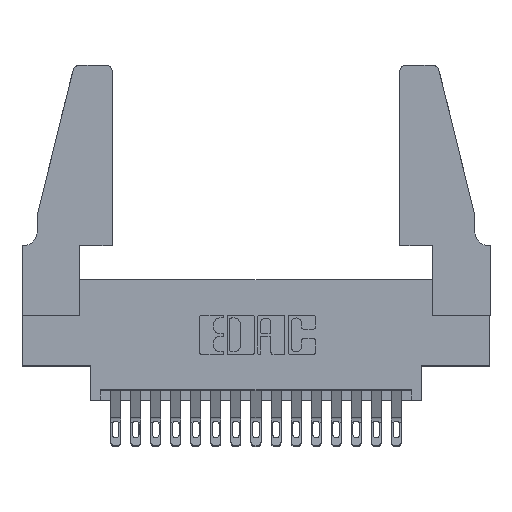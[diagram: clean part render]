
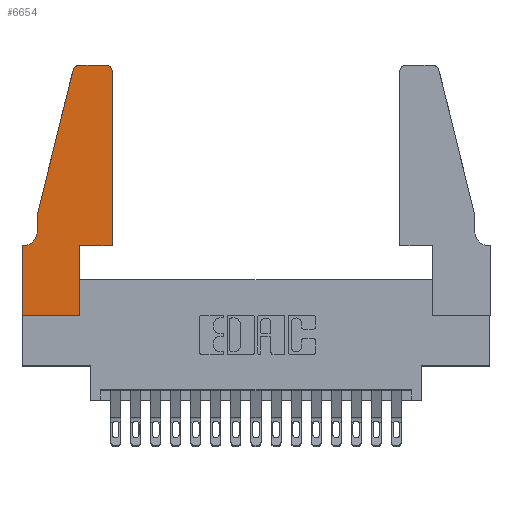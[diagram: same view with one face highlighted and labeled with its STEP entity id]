
A CAD part, top view. The second image highlights one B-rep face of the part: STEP entity #6654.
In plain terms, the highlighted planar face has unit normal (0, 0, 1).
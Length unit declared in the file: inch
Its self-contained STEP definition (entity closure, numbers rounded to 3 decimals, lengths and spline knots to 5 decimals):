
#56 = EDGE_CURVE ( 'NONE', #10528, #17273, #4938, .T. ) ;
#366 = ORIENTED_EDGE ( 'NONE', *, *, #56, .T. ) ;
#660 = CARTESIAN_POINT ( 'NONE',  ( 0.0055, 0.35, 0.37 ) ) ;
#1208 = DIRECTION ( 'NONE',  ( 1., 0., 0. ) ) ;
#1233 = VERTEX_POINT ( 'NONE', #3047 ) ;
#1381 = CARTESIAN_POINT ( 'NONE',  ( 0., 0., 0.37 ) ) ;
#1388 = LINE ( 'NONE', #16381, #8575 ) ;
#1417 = DIRECTION ( 'NONE',  ( -1., 0., 0. ) ) ;
#1424 = EDGE_CURVE ( 'NONE', #9109, #14748, #5887, .T. ) ;
#1630 = DIRECTION ( 'NONE',  ( -1., 0., 0. ) ) ;
#1920 = DIRECTION ( 'NONE',  ( -0.239, -0.971, 0. ) ) ;
#2594 = DIRECTION ( 'NONE',  ( 0., 1., 0. ) ) ;
#2750 = DIRECTION ( 'NONE',  ( 1., 0., 0. ) ) ;
#2854 = CIRCLE ( 'NONE', #13362, 0.03 ) ;
#3047 = CARTESIAN_POINT ( 'NONE',  ( 0.4505, 0.35, 0.37 ) ) ;
#3548 = EDGE_CURVE ( 'NONE', #12391, #12999, #15243, .T. ) ;
#3705 = CARTESIAN_POINT ( 'NONE',  ( 0., 0.35, 0.37 ) ) ;
#3748 = CARTESIAN_POINT ( 'NONE',  ( 0.0055, 0.42, 0.37 ) ) ;
#3931 = ORIENTED_EDGE ( 'NONE', *, *, #9454, .T. ) ;
#4114 = DIRECTION ( 'NONE',  ( 0., -1., 0. ) ) ;
#4265 = ORIENTED_EDGE ( 'NONE', *, *, #15365, .T. ) ;
#4273 = EDGE_LOOP ( 'NONE', ( #11260, #16842, #14649, #17020, #5643, #3931, #4265, #13431, #5508, #12629, #14106, #366 ) ) ;
#4326 = AXIS2_PLACEMENT_3D ( 'NONE', #6037, #16224, #4926 ) ;
#4481 = CARTESIAN_POINT ( 'NONE',  ( 0.0755, 0.5, 0.37 ) ) ;
#4529 = EDGE_CURVE ( 'NONE', #14748, #12391, #17937, .T. ) ;
#4589 = LINE ( 'NONE', #15161, #11488 ) ;
#4609 = AXIS2_PLACEMENT_3D ( 'NONE', #3748, #13409, #5184 ) ;
#4810 = VECTOR ( 'NONE', #4114, 39.37008 ) ;
#4908 = VERTEX_POINT ( 'NONE', #14956 ) ;
#4926 = DIRECTION ( 'NONE',  ( 1., 0., 0. ) ) ;
#4938 = CIRCLE ( 'NONE', #4326, 0.03 ) ;
#4985 = EDGE_CURVE ( 'NONE', #17910, #9109, #2854, .T. ) ;
#5065 = CARTESIAN_POINT ( 'NONE',  ( 0.4505, 0.35, 0.37 ) ) ;
#5077 = FACE_OUTER_BOUND ( 'NONE', #4273, .T. ) ;
#5149 = DIRECTION ( 'NONE',  ( 0., 0., 1. ) ) ;
#5184 = DIRECTION ( 'NONE',  ( -1., 0., 0. ) ) ;
#5406 = EDGE_CURVE ( 'NONE', #1233, #10528, #17472, .T. ) ;
#5456 = VECTOR ( 'NONE', #1920, 39.37008 ) ;
#5508 = ORIENTED_EDGE ( 'NONE', *, *, #14032, .T. ) ;
#5557 = CARTESIAN_POINT ( 'NONE',  ( 0.4205, 1.25, 0.37 ) ) ;
#5643 = ORIENTED_EDGE ( 'NONE', *, *, #3548, .T. ) ;
#5815 = CARTESIAN_POINT ( 'NONE',  ( 0.0755, 0.35, 0.37 ) ) ;
#5887 = LINE ( 'NONE', #7987, #5456 ) ;
#6037 = CARTESIAN_POINT ( 'NONE',  ( 0.4205, 1.22, 0.37 ) ) ;
#6654 = ADVANCED_FACE ( 'NONE', ( #5077 ), #12013, .T. ) ;
#6904 = CARTESIAN_POINT ( 'NONE',  ( 0.0755, 0.5, 0.37 ) ) ;
#7640 = VERTEX_POINT ( 'NONE', #1381 ) ;
#7987 = CARTESIAN_POINT ( 'NONE',  ( 0.0755, 0.5, 0.37 ) ) ;
#8289 = CARTESIAN_POINT ( 'NONE',  ( 0.4505, 1.22, 0.37 ) ) ;
#8575 = VECTOR ( 'NONE', #2594, 39.37008 ) ;
#8768 = CARTESIAN_POINT ( 'NONE',  ( 0.2605, 1.25, 0.37 ) ) ;
#9109 = VERTEX_POINT ( 'NONE', #17304 ) ;
#9454 = EDGE_CURVE ( 'NONE', #12999, #4908, #17019, .T. ) ;
#9646 = CARTESIAN_POINT ( 'NONE',  ( 0., 0., 0.37 ) ) ;
#9704 = CARTESIAN_POINT ( 'NONE',  ( 0.284, 1.25, 0.37 ) ) ;
#9735 = DIRECTION ( 'NONE',  ( 0., 0., 1. ) ) ;
#9878 = VECTOR ( 'NONE', #17326, 39.37008 ) ;
#10528 = VERTEX_POINT ( 'NONE', #8289 ) ;
#10578 = EDGE_CURVE ( 'NONE', #7640, #11479, #4589, .T. ) ;
#11260 = ORIENTED_EDGE ( 'NONE', *, *, #15573, .T. ) ;
#11479 = VERTEX_POINT ( 'NONE', #13975 ) ;
#11488 = VECTOR ( 'NONE', #2750, 39.37008 ) ;
#11913 = VECTOR ( 'NONE', #1630, 39.37008 ) ;
#12013 = PLANE ( 'NONE',  #17093 ) ;
#12133 = LINE ( 'NONE', #9646, #4810 ) ;
#12371 = VERTEX_POINT ( 'NONE', #17403 ) ;
#12391 = VERTEX_POINT ( 'NONE', #16114 ) ;
#12629 = ORIENTED_EDGE ( 'NONE', *, *, #13961, .T. ) ;
#12739 = DIRECTION ( 'NONE',  ( 0., -1., 0. ) ) ;
#12999 = VERTEX_POINT ( 'NONE', #660 ) ;
#13026 = VECTOR ( 'NONE', #1417, 39.37008 ) ;
#13362 = AXIS2_PLACEMENT_3D ( 'NONE', #17822, #9735, #1208 ) ;
#13409 = DIRECTION ( 'NONE',  ( 0., 0., -1. ) ) ;
#13431 = ORIENTED_EDGE ( 'NONE', *, *, #10578, .T. ) ;
#13877 = LINE ( 'NONE', #17593, #17028 ) ;
#13961 = EDGE_CURVE ( 'NONE', #12371, #1233, #13877, .T. ) ;
#13975 = CARTESIAN_POINT ( 'NONE',  ( 0.2865, 0., 0.37 ) ) ;
#14032 = EDGE_CURVE ( 'NONE', #11479, #12371, #1388, .T. ) ;
#14106 = ORIENTED_EDGE ( 'NONE', *, *, #5406, .T. ) ;
#14649 = ORIENTED_EDGE ( 'NONE', *, *, #1424, .T. ) ;
#14720 = DIRECTION ( 'NONE',  ( 1., 0., 0. ) ) ;
#14748 = VERTEX_POINT ( 'NONE', #6904 ) ;
#14908 = DIRECTION ( 'NONE',  ( 1., 0., 0. ) ) ;
#14956 = CARTESIAN_POINT ( 'NONE',  ( 0., 0.35, 0.37 ) ) ;
#15161 = CARTESIAN_POINT ( 'NONE',  ( 0., 0., 0.37 ) ) ;
#15243 = CIRCLE ( 'NONE', #4609, 0.07 ) ;
#15365 = EDGE_CURVE ( 'NONE', #4908, #7640, #12133, .T. ) ;
#15573 = EDGE_CURVE ( 'NONE', #17273, #17910, #15917, .T. ) ;
#15917 = LINE ( 'NONE', #8768, #11913 ) ;
#16114 = CARTESIAN_POINT ( 'NONE',  ( 0.0755, 0.42, 0.37 ) ) ;
#16224 = DIRECTION ( 'NONE',  ( 0., 0., 1. ) ) ;
#16381 = CARTESIAN_POINT ( 'NONE',  ( 0.2865, 0.35, 0.37 ) ) ;
#16670 = VECTOR ( 'NONE', #12739, 39.37008 ) ;
#16842 = ORIENTED_EDGE ( 'NONE', *, *, #4985, .T. ) ;
#17019 = LINE ( 'NONE', #5815, #13026 ) ;
#17020 = ORIENTED_EDGE ( 'NONE', *, *, #4529, .T. ) ;
#17028 = VECTOR ( 'NONE', #14908, 39.37008 ) ;
#17093 = AXIS2_PLACEMENT_3D ( 'NONE', #3705, #5149, #14720 ) ;
#17273 = VERTEX_POINT ( 'NONE', #5557 ) ;
#17304 = CARTESIAN_POINT ( 'NONE',  ( 0.25487, 1.22718, 0.37 ) ) ;
#17326 = DIRECTION ( 'NONE',  ( 0., 1., 0. ) ) ;
#17403 = CARTESIAN_POINT ( 'NONE',  ( 0.2865, 0.35, 0.37 ) ) ;
#17472 = LINE ( 'NONE', #5065, #9878 ) ;
#17593 = CARTESIAN_POINT ( 'NONE',  ( 0.4505, 0.35, 0.37 ) ) ;
#17822 = CARTESIAN_POINT ( 'NONE',  ( 0.284, 1.22, 0.37 ) ) ;
#17910 = VERTEX_POINT ( 'NONE', #9704 ) ;
#17937 = LINE ( 'NONE', #4481, #16670 ) ;
